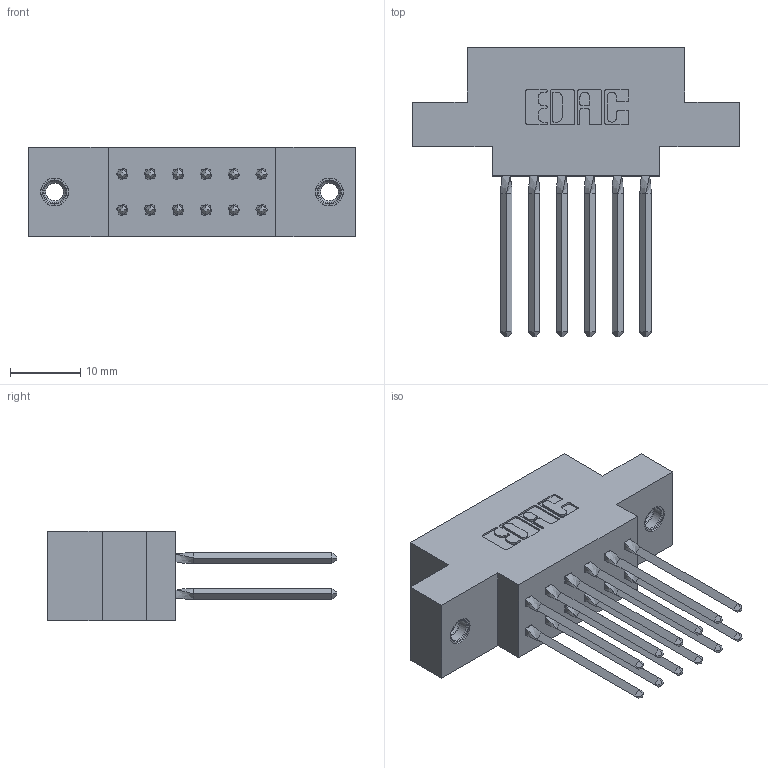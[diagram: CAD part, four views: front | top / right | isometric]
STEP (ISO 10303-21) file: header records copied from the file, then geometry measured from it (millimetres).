
FILE_DESCRIPTION (( 'STEP AP203' ), '1' );
FILE_NAME ('317-012-543-807.STEP', '2020-02-27T14:16:32', ( '' ), ( '' ), 'SwSTEP 2.0', 'SolidWorks 2016', '' );
FILE_SCHEMA (( 'CONFIG_CONTROL_DESIGN' ));
Length unit declared in the file: inch
Products named in the file (4): 345-250-001_345-250-005-103; 317-290-001_543; 317-012-543-807; 317 Part_.156 Dia - TI
Assembly tree (15 placements, depth 2):
  317-012-543-807
    317 Part_.156 Dia - TI
    317-290-001_543  x12
    345-250-001_345-250-005-103  x2
Bounding box: 46.48 x 41.15 x 12.7 mm (x, y, z)
Volume: 6630.1 mm3; surface area: 8681.8 mm2
Topology: 15 solids, 15 shells, 1230 faces, 3375 edges, 2174 vertices
Faces by surface type: plane 966, cylinder 200, bspline 48, cone 12, torus 4
Entity records: 14881 total; most frequent: CARTESIAN_POINT 2978, ORIENTED_EDGE 2470, DIRECTION 2107, EDGE_CURVE 1235, LINE 959, VECTOR 959, VERTEX_POINT 813, AXIS2_PLACEMENT_3D 574
